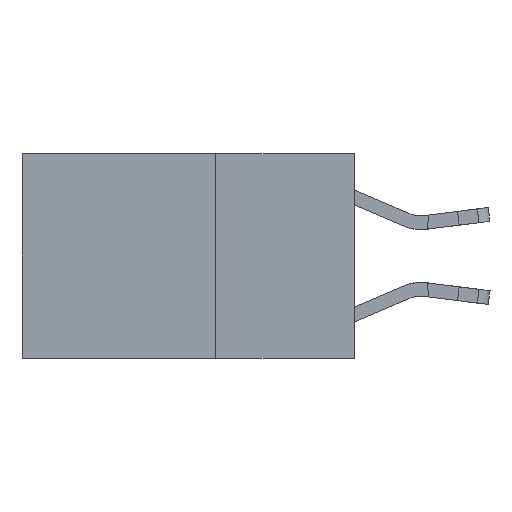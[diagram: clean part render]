
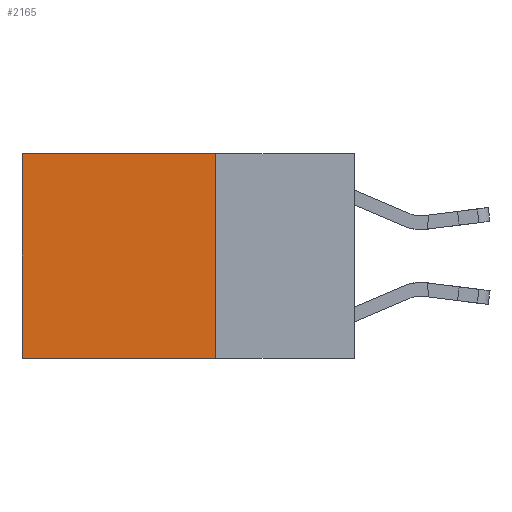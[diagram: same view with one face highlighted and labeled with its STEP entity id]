
A CAD part, left-side view. The second image highlights one B-rep face of the part: STEP entity #2165.
In plain terms, the highlighted planar face has unit normal (-1, 0, 0).
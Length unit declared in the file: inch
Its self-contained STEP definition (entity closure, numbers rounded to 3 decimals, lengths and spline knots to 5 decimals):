
#310 = LINE ( 'NONE', #8823, #14333 ) ;
#943 = ORIENTED_EDGE ( 'NONE', *, *, #11036, .T. ) ;
#2144 = DIRECTION ( 'NONE',  ( 0., 0., -1. ) ) ;
#2165 = ADVANCED_FACE ( 'NONE', ( #12422 ), #8915, .F. ) ;
#2430 = ORIENTED_EDGE ( 'NONE', *, *, #16747, .F. ) ;
#2485 = CARTESIAN_POINT ( 'NONE',  ( 0.2625, 0.25, 0. ) ) ;
#3042 = ORIENTED_EDGE ( 'NONE', *, *, #9421, .F. ) ;
#4018 = VERTEX_POINT ( 'NONE', #14175 ) ;
#4427 = CARTESIAN_POINT ( 'NONE',  ( 0.2625, 0.25, -0.37 ) ) ;
#5047 = CARTESIAN_POINT ( 'NONE',  ( 0.2625, 0.25, -0.37 ) ) ;
#6796 = CARTESIAN_POINT ( 'NONE',  ( 0.2625, 0.6, 0. ) ) ;
#7534 = CARTESIAN_POINT ( 'NONE',  ( 0.2625, 0.25, 0. ) ) ;
#8096 = VECTOR ( 'NONE', #8104, 39.37008 ) ;
#8104 = DIRECTION ( 'NONE',  ( 0., 0., -1. ) ) ;
#8424 = VERTEX_POINT ( 'NONE', #5047 ) ;
#8823 = CARTESIAN_POINT ( 'NONE',  ( 0.2625, 0.25, 0. ) ) ;
#8915 = PLANE ( 'NONE',  #15995 ) ;
#9421 = EDGE_CURVE ( 'NONE', #10902, #8424, #310, .T. ) ;
#10010 = VECTOR ( 'NONE', #14269, 39.37008 ) ;
#10197 = CARTESIAN_POINT ( 'NONE',  ( 0.2625, 0.25, 0. ) ) ;
#10213 = DIRECTION ( 'NONE',  ( 0., 0., -1. ) ) ;
#10310 = DIRECTION ( 'NONE',  ( 1., 0., 0. ) ) ;
#10321 = ORIENTED_EDGE ( 'NONE', *, *, #12006, .T. ) ;
#10902 = VERTEX_POINT ( 'NONE', #2485 ) ;
#11036 = EDGE_CURVE ( 'NONE', #11165, #4018, #15320, .T. ) ;
#11165 = VERTEX_POINT ( 'NONE', #13891 ) ;
#11589 = VECTOR ( 'NONE', #12606, 39.37008 ) ;
#11989 = LINE ( 'NONE', #4427, #11589 ) ;
#12006 = EDGE_CURVE ( 'NONE', #10902, #11165, #17199, .T. ) ;
#12422 = FACE_OUTER_BOUND ( 'NONE', #12522, .T. ) ;
#12522 = EDGE_LOOP ( 'NONE', ( #943, #2430, #3042, #10321 ) ) ;
#12606 = DIRECTION ( 'NONE',  ( 0., 1., 0. ) ) ;
#13891 = CARTESIAN_POINT ( 'NONE',  ( 0.2625, 0.6, 0. ) ) ;
#14175 = CARTESIAN_POINT ( 'NONE',  ( 0.2625, 0.6, -0.37 ) ) ;
#14269 = DIRECTION ( 'NONE',  ( 0., 1., 0. ) ) ;
#14333 = VECTOR ( 'NONE', #10213, 39.37008 ) ;
#15320 = LINE ( 'NONE', #6796, #8096 ) ;
#15995 = AXIS2_PLACEMENT_3D ( 'NONE', #7534, #10310, #2144 ) ;
#16747 = EDGE_CURVE ( 'NONE', #8424, #4018, #11989, .T. ) ;
#17199 = LINE ( 'NONE', #10197, #10010 ) ;
